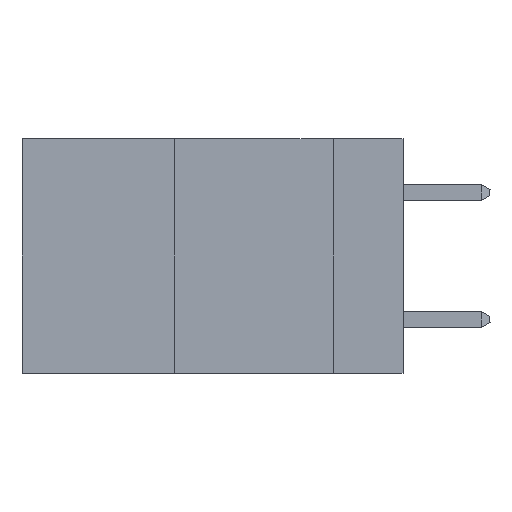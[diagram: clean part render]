
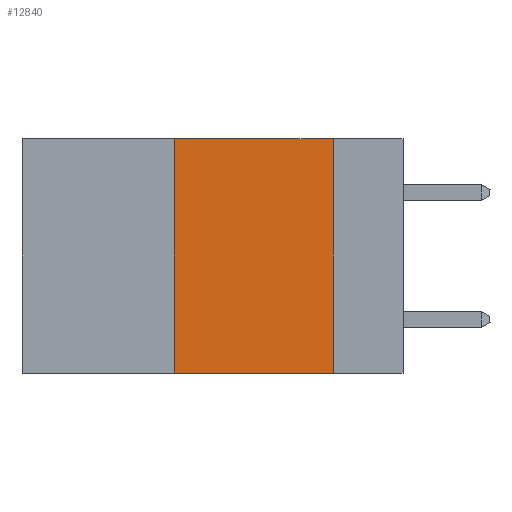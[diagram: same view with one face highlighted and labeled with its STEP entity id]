
A CAD part, left-side view. The second image highlights one B-rep face of the part: STEP entity #12840.
In plain terms, the highlighted planar face has unit normal (-1, 0, 0).
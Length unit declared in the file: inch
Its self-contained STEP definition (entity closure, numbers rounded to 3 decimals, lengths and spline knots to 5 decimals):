
#1905 = CARTESIAN_POINT ( 'NONE',  ( 0., 0.36, 0. ) ) ;
#2144 = DIRECTION ( 'NONE',  ( 1., 0., 0. ) ) ;
#3429 = VERTEX_POINT ( 'NONE', #29116 ) ;
#3672 = LINE ( 'NONE', #13574, #11052 ) ;
#5654 = EDGE_CURVE ( 'NONE', #3429, #22776, #3672, .T. ) ;
#5753 = LINE ( 'NONE', #16000, #18007 ) ;
#7602 = VECTOR ( 'NONE', #22198, 39.37008 ) ;
#8710 = CARTESIAN_POINT ( 'NONE',  ( 0., 0.11, 0. ) ) ;
#10579 = DIRECTION ( 'NONE',  ( 0., 0., 1. ) ) ;
#11052 = VECTOR ( 'NONE', #10579, 39.37008 ) ;
#12840 = ADVANCED_FACE ( 'NONE', ( #39979 ), #20974, .F. ) ;
#13178 = AXIS2_PLACEMENT_3D ( 'NONE', #39754, #2144, #24178 ) ;
#13574 = CARTESIAN_POINT ( 'NONE',  ( 0., 0.36, 0. ) ) ;
#13618 = CARTESIAN_POINT ( 'NONE',  ( 0., 0.6, -0.37 ) ) ;
#13877 = LINE ( 'NONE', #13618, #25266 ) ;
#16000 = CARTESIAN_POINT ( 'NONE',  ( 0., 0.6, 0. ) ) ;
#16779 = ORIENTED_EDGE ( 'NONE', *, *, #35746, .T. ) ;
#16952 = CARTESIAN_POINT ( 'NONE',  ( 0., 0.11, 0. ) ) ;
#17873 = CARTESIAN_POINT ( 'NONE',  ( 0., 0.11, -0.37 ) ) ;
#18007 = VECTOR ( 'NONE', #31837, 39.37008 ) ;
#19825 = DIRECTION ( 'NONE',  ( 0., -1., 0. ) ) ;
#20974 = PLANE ( 'NONE',  #13178 ) ;
#22198 = DIRECTION ( 'NONE',  ( 0., 0., -1. ) ) ;
#22776 = VERTEX_POINT ( 'NONE', #1905 ) ;
#24178 = DIRECTION ( 'NONE',  ( 0., 0., -1. ) ) ;
#24233 = ORIENTED_EDGE ( 'NONE', *, *, #27677, .F. ) ;
#25266 = VECTOR ( 'NONE', #19825, 39.37008 ) ;
#27677 = EDGE_CURVE ( 'NONE', #22776, #32243, #5753, .T. ) ;
#28199 = ORIENTED_EDGE ( 'NONE', *, *, #5654, .F. ) ;
#28718 = EDGE_CURVE ( 'NONE', #32243, #30489, #30244, .T. ) ;
#29116 = CARTESIAN_POINT ( 'NONE',  ( 0., 0.36, -0.37 ) ) ;
#30244 = LINE ( 'NONE', #8710, #7602 ) ;
#30489 = VERTEX_POINT ( 'NONE', #17873 ) ;
#31837 = DIRECTION ( 'NONE',  ( 0., -1., 0. ) ) ;
#32243 = VERTEX_POINT ( 'NONE', #16952 ) ;
#33915 = ORIENTED_EDGE ( 'NONE', *, *, #28718, .F. ) ;
#35746 = EDGE_CURVE ( 'NONE', #3429, #30489, #13877, .T. ) ;
#39381 = EDGE_LOOP ( 'NONE', ( #33915, #24233, #28199, #16779 ) ) ;
#39754 = CARTESIAN_POINT ( 'NONE',  ( 0., 0.6, 0. ) ) ;
#39979 = FACE_OUTER_BOUND ( 'NONE', #39381, .T. ) ;
